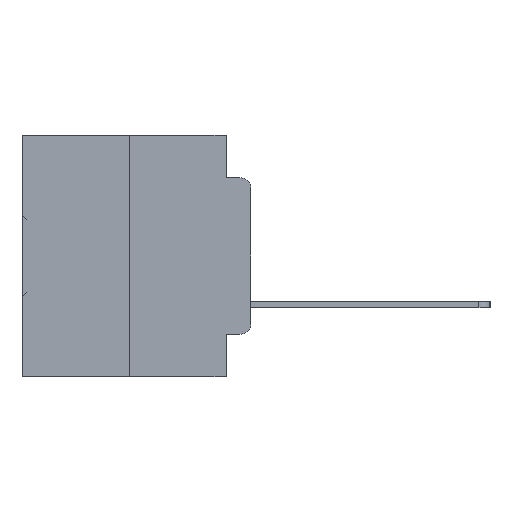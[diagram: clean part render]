
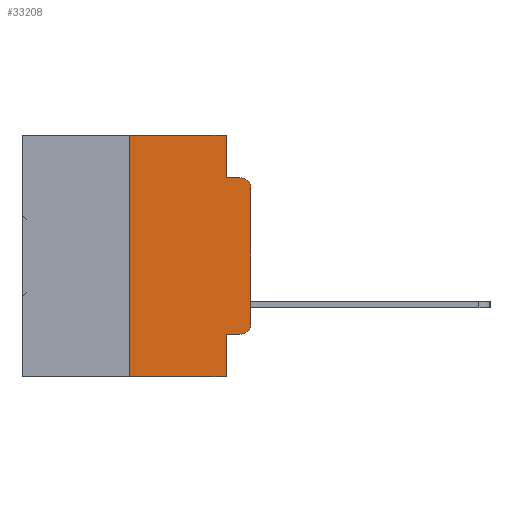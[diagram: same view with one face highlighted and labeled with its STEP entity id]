
A CAD part, left-side view. The second image highlights one B-rep face of the part: STEP entity #33208.
In plain terms, the highlighted planar face has unit normal (-1, 0, 0).
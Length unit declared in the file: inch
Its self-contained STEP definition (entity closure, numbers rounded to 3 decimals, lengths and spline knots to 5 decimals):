
#558 = EDGE_CURVE ( 'NONE', #30630, #18515, #24195, .T. ) ;
#573 = EDGE_CURVE ( 'NONE', #32379, #4764, #24543, .T. ) ;
#836 = DIRECTION ( 'NONE',  ( 0., -1., 0. ) ) ;
#1021 = LINE ( 'NONE', #31880, #11597 ) ;
#1856 = CARTESIAN_POINT ( 'NONE',  ( 0., 0.02, -0.1085 ) ) ;
#2069 = CARTESIAN_POINT ( 'NONE',  ( 0., 0.051, 0. ) ) ;
#2372 = CARTESIAN_POINT ( 'NONE',  ( 0., 0.051, -0.0885 ) ) ;
#2568 = VECTOR ( 'NONE', #21276, 39.37008 ) ;
#3654 = VECTOR ( 'NONE', #13236, 39.37008 ) ;
#4003 = LINE ( 'NONE', #9045, #2568 ) ;
#4144 = CARTESIAN_POINT ( 'NONE',  ( 0., 0.051, 0. ) ) ;
#4764 = VERTEX_POINT ( 'NONE', #31116 ) ;
#6012 = VERTEX_POINT ( 'NONE', #2069 ) ;
#6203 = EDGE_LOOP ( 'NONE', ( #7909, #10340, #16070, #26796, #8772, #10147, #19016, #11881, #30592, #26402 ) ) ;
#6486 = CARTESIAN_POINT ( 'NONE',  ( 0., 0.473, 0. ) ) ;
#7207 = DIRECTION ( 'NONE',  ( 0., 0., -1. ) ) ;
#7249 = EDGE_CURVE ( 'NONE', #17224, #24874, #4003, .T. ) ;
#7909 = ORIENTED_EDGE ( 'NONE', *, *, #7249, .T. ) ;
#7979 = LINE ( 'NONE', #16135, #33362 ) ;
#8019 = DIRECTION ( 'NONE',  ( -1., 0., 0. ) ) ;
#8772 = ORIENTED_EDGE ( 'NONE', *, *, #23929, .F. ) ;
#8882 = DIRECTION ( 'NONE',  ( 0., 0., -1. ) ) ;
#9045 = CARTESIAN_POINT ( 'NONE',  ( 0., 0., 0. ) ) ;
#10147 = ORIENTED_EDGE ( 'NONE', *, *, #573, .F. ) ;
#10340 = ORIENTED_EDGE ( 'NONE', *, *, #28914, .T. ) ;
#10371 = CARTESIAN_POINT ( 'NONE',  ( 0., 0., -0.1085 ) ) ;
#10455 = CARTESIAN_POINT ( 'NONE',  ( 0., 0.25, -0.5 ) ) ;
#11597 = VECTOR ( 'NONE', #836, 39.37008 ) ;
#11881 = ORIENTED_EDGE ( 'NONE', *, *, #558, .F. ) ;
#12850 = DIRECTION ( 'NONE',  ( 0., -1., 0. ) ) ;
#13236 = DIRECTION ( 'NONE',  ( 0., 0., 1. ) ) ;
#13369 = CARTESIAN_POINT ( 'NONE',  ( 0., 0.051, -0.4115 ) ) ;
#14075 = DIRECTION ( 'NONE',  ( 0., -1., 0. ) ) ;
#15331 = VECTOR ( 'NONE', #12850, 39.37008 ) ;
#16028 = AXIS2_PLACEMENT_3D ( 'NONE', #1856, #8019, #19329 ) ;
#16070 = ORIENTED_EDGE ( 'NONE', *, *, #29439, .F. ) ;
#16135 = CARTESIAN_POINT ( 'NONE',  ( 0., 0.051, 0. ) ) ;
#16163 = CARTESIAN_POINT ( 'NONE',  ( 0., 0.473, -0.5 ) ) ;
#16297 = CARTESIAN_POINT ( 'NONE',  ( 0., 0.051, -0.4115 ) ) ;
#16803 = AXIS2_PLACEMENT_3D ( 'NONE', #6486, #24281, #7207 ) ;
#17224 = VERTEX_POINT ( 'NONE', #29513 ) ;
#18515 = VERTEX_POINT ( 'NONE', #25073 ) ;
#19016 = ORIENTED_EDGE ( 'NONE', *, *, #27000, .T. ) ;
#19329 = DIRECTION ( 'NONE',  ( 0., 0., -1. ) ) ;
#19807 = CARTESIAN_POINT ( 'NONE',  ( 0., 0.02, -0.3915 ) ) ;
#19839 = DIRECTION ( 'NONE',  ( 0., -1., 0. ) ) ;
#20024 = LINE ( 'NONE', #2372, #24935 ) ;
#20809 = VERTEX_POINT ( 'NONE', #29659 ) ;
#21276 = DIRECTION ( 'NONE',  ( 0., 0., 1. ) ) ;
#21324 = FACE_OUTER_BOUND ( 'NONE', #6203, .T. ) ;
#22165 = AXIS2_PLACEMENT_3D ( 'NONE', #19807, #25373, #8882 ) ;
#22435 = EDGE_CURVE ( 'NONE', #30630, #26350, #27636, .T. ) ;
#23102 = VERTEX_POINT ( 'NONE', #23340 ) ;
#23340 = CARTESIAN_POINT ( 'NONE',  ( 0., 0.051, -0.0885 ) ) ;
#23929 = EDGE_CURVE ( 'NONE', #4764, #6012, #1021, .T. ) ;
#24195 = LINE ( 'NONE', #4144, #34494 ) ;
#24281 = DIRECTION ( 'NONE',  ( 1., 0., 0. ) ) ;
#24543 = LINE ( 'NONE', #36235, #3654 ) ;
#24874 = VERTEX_POINT ( 'NONE', #10371 ) ;
#24935 = VECTOR ( 'NONE', #19839, 39.37008 ) ;
#25073 = CARTESIAN_POINT ( 'NONE',  ( 0., 0.051, -0.5 ) ) ;
#25373 = DIRECTION ( 'NONE',  ( -1., 0., 0. ) ) ;
#26350 = VERTEX_POINT ( 'NONE', #30608 ) ;
#26402 = ORIENTED_EDGE ( 'NONE', *, *, #33425, .T. ) ;
#26795 = DIRECTION ( 'NONE',  ( 0., 0., -1. ) ) ;
#26796 = ORIENTED_EDGE ( 'NONE', *, *, #30651, .F. ) ;
#27000 = EDGE_CURVE ( 'NONE', #32379, #18515, #32882, .T. ) ;
#27104 = DIRECTION ( 'NONE',  ( 0., 0., -1. ) ) ;
#27636 = LINE ( 'NONE', #16297, #36566 ) ;
#28914 = EDGE_CURVE ( 'NONE', #24874, #20809, #32059, .T. ) ;
#29439 = EDGE_CURVE ( 'NONE', #23102, #20809, #20024, .T. ) ;
#29513 = CARTESIAN_POINT ( 'NONE',  ( 0., 0., -0.3915 ) ) ;
#29659 = CARTESIAN_POINT ( 'NONE',  ( 0., 0.02, -0.0885 ) ) ;
#30592 = ORIENTED_EDGE ( 'NONE', *, *, #22435, .T. ) ;
#30608 = CARTESIAN_POINT ( 'NONE',  ( 0., 0.02, -0.4115 ) ) ;
#30630 = VERTEX_POINT ( 'NONE', #13369 ) ;
#30651 = EDGE_CURVE ( 'NONE', #6012, #23102, #7979, .T. ) ;
#31116 = CARTESIAN_POINT ( 'NONE',  ( 0., 0.25, 0. ) ) ;
#31880 = CARTESIAN_POINT ( 'NONE',  ( 0., 0.473, 0. ) ) ;
#32059 = CIRCLE ( 'NONE', #16028, 0.02 ) ;
#32379 = VERTEX_POINT ( 'NONE', #10455 ) ;
#32635 = PLANE ( 'NONE',  #16803 ) ;
#32882 = LINE ( 'NONE', #16163, #15331 ) ;
#33208 = ADVANCED_FACE ( 'NONE', ( #21324 ), #32635, .F. ) ;
#33362 = VECTOR ( 'NONE', #27104, 39.37008 ) ;
#33418 = CIRCLE ( 'NONE', #22165, 0.02 ) ;
#33425 = EDGE_CURVE ( 'NONE', #26350, #17224, #33418, .T. ) ;
#34494 = VECTOR ( 'NONE', #26795, 39.37008 ) ;
#36235 = CARTESIAN_POINT ( 'NONE',  ( 0., 0.25, 0. ) ) ;
#36566 = VECTOR ( 'NONE', #14075, 39.37008 ) ;
